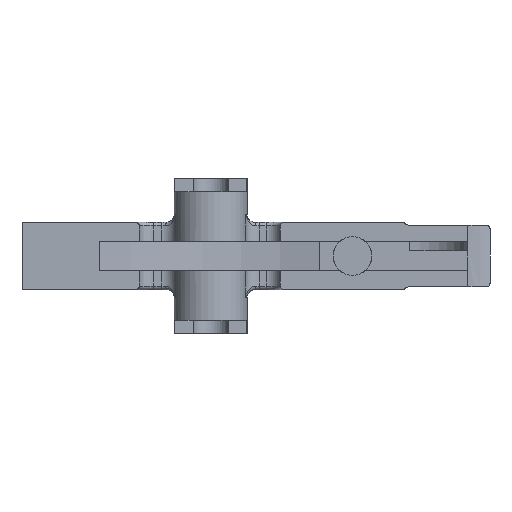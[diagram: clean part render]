
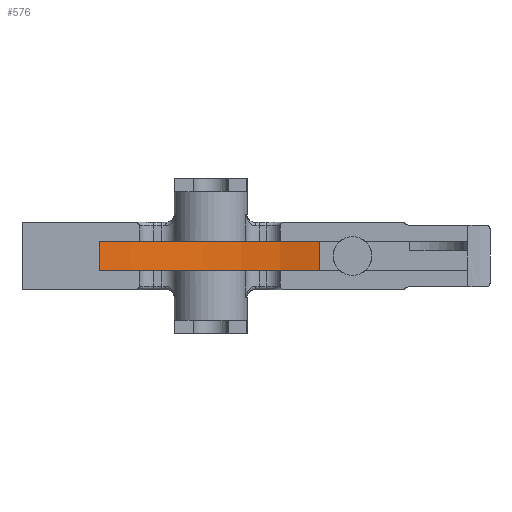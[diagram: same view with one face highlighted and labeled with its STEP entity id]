
A CAD part, front view. The second image highlights one B-rep face of the part: STEP entity #576.
In plain terms, the highlighted cylindrical face has radius 25.364 mm (diameter 50.729 mm), a partial arc.
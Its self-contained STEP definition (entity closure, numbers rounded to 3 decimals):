
#396 = VERTEX_POINT ( 'NONE', #6665 ) ;
#541 = AXIS2_PLACEMENT_3D ( 'NONE', #1962, #4668, #1397 ) ;
#576 = ADVANCED_FACE ( 'NONE', ( #4632 ), #1928, .F. ) ;
#1144 = DIRECTION ( 'NONE',  ( 0., 0., 1. ) ) ;
#1217 = CARTESIAN_POINT ( 'NONE',  ( 21.037, -2.195, -1.587 ) ) ;
#1397 = DIRECTION ( 'NONE',  ( 1., 0., 0. ) ) ;
#1503 = DIRECTION ( 'NONE',  ( -1., 0., 0. ) ) ;
#1664 = EDGE_CURVE ( 'NONE', #5710, #2125, #5957, .T. ) ;
#1828 = CARTESIAN_POINT ( 'NONE',  ( 21.037, -2.195, 1.587 ) ) ;
#1928 = CYLINDRICAL_SURFACE ( 'NONE', #541, 25.364 ) ;
#1962 = CARTESIAN_POINT ( 'NONE',  ( 14.696, -26.753, -1.587 ) ) ;
#2019 = DIRECTION ( 'NONE',  ( 0., 0., 1. ) ) ;
#2125 = VERTEX_POINT ( 'NONE', #1828 ) ;
#2242 = EDGE_CURVE ( 'NONE', #2125, #4493, #4536, .T. ) ;
#2750 = CIRCLE ( 'NONE', #6671, 25.364 ) ;
#2752 = EDGE_LOOP ( 'NONE', ( #4354, #5389, #6367, #5197 ) ) ;
#2985 = AXIS2_PLACEMENT_3D ( 'NONE', #3839, #4854, #5912 ) ;
#3181 = CARTESIAN_POINT ( 'NONE',  ( 14.696, -26.753, -1.587 ) ) ;
#3279 = VECTOR ( 'NONE', #2019, 1000. ) ;
#3839 = CARTESIAN_POINT ( 'NONE',  ( 14.696, -26.753, 1.587 ) ) ;
#4218 = CARTESIAN_POINT ( 'NONE',  ( -2.891, -8.476, 1.587 ) ) ;
#4354 = ORIENTED_EDGE ( 'NONE', *, *, #2242, .T. ) ;
#4468 = EDGE_CURVE ( 'NONE', #5710, #396, #2750, .T. ) ;
#4493 = VERTEX_POINT ( 'NONE', #4218 ) ;
#4536 = CIRCLE ( 'NONE', #2985, 25.364 ) ;
#4632 = FACE_OUTER_BOUND ( 'NONE', #2752, .T. ) ;
#4668 = DIRECTION ( 'NONE',  ( 0., 0., 1. ) ) ;
#4854 = DIRECTION ( 'NONE',  ( 0., 0., 1. ) ) ;
#5197 = ORIENTED_EDGE ( 'NONE', *, *, #1664, .T. ) ;
#5229 = VECTOR ( 'NONE', #1144, 1000. ) ;
#5289 = CARTESIAN_POINT ( 'NONE',  ( -2.891, -8.476, -1.587 ) ) ;
#5389 = ORIENTED_EDGE ( 'NONE', *, *, #6201, .F. ) ;
#5710 = VERTEX_POINT ( 'NONE', #6599 ) ;
#5912 = DIRECTION ( 'NONE',  ( -1., 0., 0. ) ) ;
#5957 = LINE ( 'NONE', #1217, #5229 ) ;
#6201 = EDGE_CURVE ( 'NONE', #396, #4493, #6941, .T. ) ;
#6367 = ORIENTED_EDGE ( 'NONE', *, *, #4468, .F. ) ;
#6404 = DIRECTION ( 'NONE',  ( 0., 0., 1. ) ) ;
#6599 = CARTESIAN_POINT ( 'NONE',  ( 21.037, -2.195, -1.587 ) ) ;
#6665 = CARTESIAN_POINT ( 'NONE',  ( -2.891, -8.476, -1.587 ) ) ;
#6671 = AXIS2_PLACEMENT_3D ( 'NONE', #3181, #6404, #1503 ) ;
#6941 = LINE ( 'NONE', #5289, #3279 ) ;
